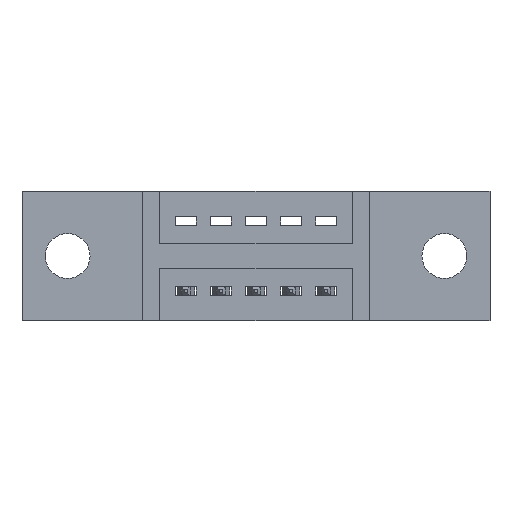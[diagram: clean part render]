
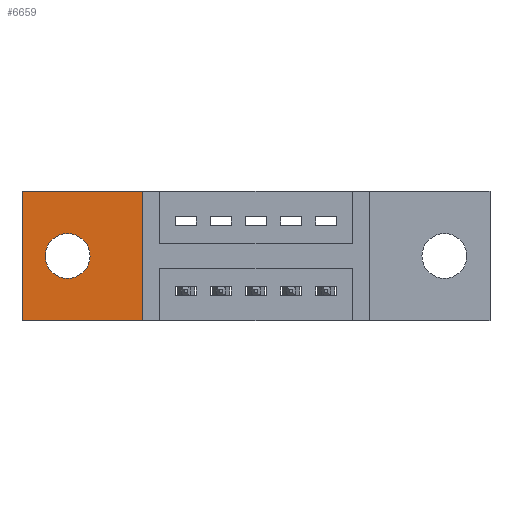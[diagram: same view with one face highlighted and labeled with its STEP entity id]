
A CAD part, front view. The second image highlights one B-rep face of the part: STEP entity #6659.
In plain terms, the highlighted planar face has unit normal (0, -1, 0).
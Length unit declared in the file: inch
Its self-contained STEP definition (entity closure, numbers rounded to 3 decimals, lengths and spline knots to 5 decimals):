
#150 = ORIENTED_EDGE ( 'NONE', *, *, #2305, .T. ) ;
#529 = ORIENTED_EDGE ( 'NONE', *, *, #5776, .T. ) ;
#692 = VERTEX_POINT ( 'NONE', #4564 ) ;
#706 = DIRECTION ( 'NONE',  ( 0., -1., 0. ) ) ;
#754 = CARTESIAN_POINT ( 'NONE',  ( 0.13, 0.17, -0.185 ) ) ;
#964 = ORIENTED_EDGE ( 'NONE', *, *, #8566, .T. ) ;
#1161 = VECTOR ( 'NONE', #4287, 39.37008 ) ;
#1389 = EDGE_CURVE ( 'NONE', #692, #3086, #3044, .T. ) ;
#1494 = LINE ( 'NONE', #5458, #4117 ) ;
#1723 = CARTESIAN_POINT ( 'NONE',  ( 0.13, 0.17, -0.249 ) ) ;
#1757 = ORIENTED_EDGE ( 'NONE', *, *, #4725, .F. ) ;
#1772 = VERTEX_POINT ( 'NONE', #8324 ) ;
#1931 = AXIS2_PLACEMENT_3D ( 'NONE', #4230, #706, #8790 ) ;
#2270 = ORIENTED_EDGE ( 'NONE', *, *, #3288, .T. ) ;
#2305 = EDGE_CURVE ( 'NONE', #1772, #3496, #5191, .T. ) ;
#2719 = CARTESIAN_POINT ( 'NONE',  ( 0., 0.17, -0.37 ) ) ;
#2968 = PLANE ( 'NONE',  #3745 ) ;
#3044 = CIRCLE ( 'NONE', #8417, 0.064 ) ;
#3086 = VERTEX_POINT ( 'NONE', #1723 ) ;
#3288 = EDGE_CURVE ( 'NONE', #3760, #4992, #4290, .T. ) ;
#3298 = CARTESIAN_POINT ( 'NONE',  ( 0.3425, 0.17, 0. ) ) ;
#3309 = LINE ( 'NONE', #3566, #6512 ) ;
#3496 = VERTEX_POINT ( 'NONE', #5626 ) ;
#3566 = CARTESIAN_POINT ( 'NONE',  ( 0., 0.17, -0.37 ) ) ;
#3578 = DIRECTION ( 'NONE',  ( 1., 0., 0. ) ) ;
#3745 = AXIS2_PLACEMENT_3D ( 'NONE', #2719, #5199, #7002 ) ;
#3760 = VERTEX_POINT ( 'NONE', #4245 ) ;
#3962 = DIRECTION ( 'NONE',  ( 0., -1., 0. ) ) ;
#4117 = VECTOR ( 'NONE', #6088, 39.37008 ) ;
#4230 = CARTESIAN_POINT ( 'NONE',  ( 0.13, 0.17, -0.185 ) ) ;
#4245 = CARTESIAN_POINT ( 'NONE',  ( 0.3425, 0.17, -0.37 ) ) ;
#4250 = DIRECTION ( 'NONE',  ( 0., 0., 1. ) ) ;
#4285 = FACE_OUTER_BOUND ( 'NONE', #5930, .T. ) ;
#4287 = DIRECTION ( 'NONE',  ( 0., 0., -1. ) ) ;
#4290 = LINE ( 'NONE', #7023, #7456 ) ;
#4564 = CARTESIAN_POINT ( 'NONE',  ( 0.13, 0.17, -0.121 ) ) ;
#4725 = EDGE_CURVE ( 'NONE', #3086, #692, #8448, .T. ) ;
#4992 = VERTEX_POINT ( 'NONE', #3298 ) ;
#5191 = LINE ( 'NONE', #7853, #1161 ) ;
#5199 = DIRECTION ( 'NONE',  ( 0., -1., 0. ) ) ;
#5267 = ORIENTED_EDGE ( 'NONE', *, *, #1389, .F. ) ;
#5458 = CARTESIAN_POINT ( 'NONE',  ( 0., 0.17, 0. ) ) ;
#5541 = DIRECTION ( 'NONE',  ( 0., 0., -1. ) ) ;
#5626 = CARTESIAN_POINT ( 'NONE',  ( 0., 0.17, -0.37 ) ) ;
#5776 = EDGE_CURVE ( 'NONE', #3496, #3760, #3309, .T. ) ;
#5930 = EDGE_LOOP ( 'NONE', ( #150, #529, #2270, #964 ) ) ;
#6088 = DIRECTION ( 'NONE',  ( -1., 0., 0. ) ) ;
#6512 = VECTOR ( 'NONE', #3578, 39.37008 ) ;
#6597 = EDGE_LOOP ( 'NONE', ( #5267, #1757 ) ) ;
#6659 = ADVANCED_FACE ( 'NONE', ( #7454, #4285 ), #2968, .T. ) ;
#7002 = DIRECTION ( 'NONE',  ( 0., 0., -1. ) ) ;
#7023 = CARTESIAN_POINT ( 'NONE',  ( 0.3425, 0.17, 0. ) ) ;
#7454 = FACE_BOUND ( 'NONE', #6597, .T. ) ;
#7456 = VECTOR ( 'NONE', #4250, 39.37008 ) ;
#7853 = CARTESIAN_POINT ( 'NONE',  ( 0., 0.17, 0. ) ) ;
#8324 = CARTESIAN_POINT ( 'NONE',  ( 0., 0.17, 0. ) ) ;
#8417 = AXIS2_PLACEMENT_3D ( 'NONE', #754, #3962, #5541 ) ;
#8448 = CIRCLE ( 'NONE', #1931, 0.064 ) ;
#8566 = EDGE_CURVE ( 'NONE', #4992, #1772, #1494, .T. ) ;
#8790 = DIRECTION ( 'NONE',  ( 0., 0., -1. ) ) ;
